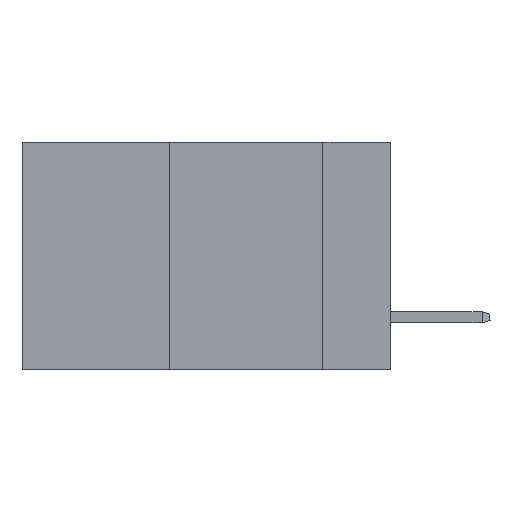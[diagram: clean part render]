
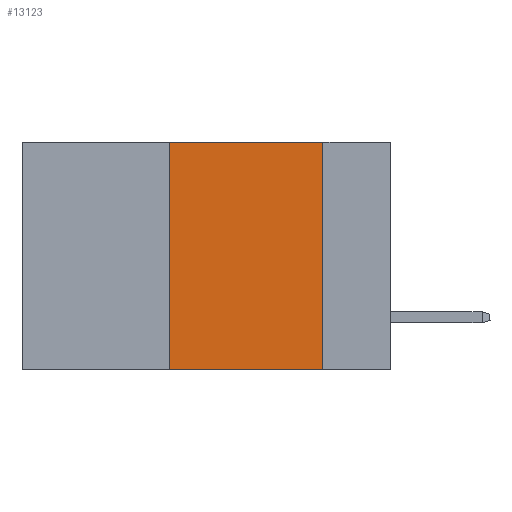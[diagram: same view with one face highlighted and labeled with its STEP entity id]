
A CAD part, left-side view. The second image highlights one B-rep face of the part: STEP entity #13123.
In plain terms, the highlighted planar face has unit normal (-1, 0, 0).
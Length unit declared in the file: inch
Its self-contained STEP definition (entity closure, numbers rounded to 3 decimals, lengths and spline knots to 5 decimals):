
#54 = ORIENTED_EDGE ( 'NONE', *, *, #2807, .F. ) ;
#209 = ORIENTED_EDGE ( 'NONE', *, *, #2925, .T. ) ;
#1054 = VERTEX_POINT ( 'NONE', #7221 ) ;
#1187 = EDGE_CURVE ( 'NONE', #2343, #9184, #7537, .T. ) ;
#1325 = DIRECTION ( 'NONE',  ( 0., -1., 0. ) ) ;
#1524 = CARTESIAN_POINT ( 'NONE',  ( 0., 0.36, 0. ) ) ;
#2074 = CARTESIAN_POINT ( 'NONE',  ( 0., 0.6, 0. ) ) ;
#2343 = VERTEX_POINT ( 'NONE', #8081 ) ;
#2496 = FACE_OUTER_BOUND ( 'NONE', #5296, .T. ) ;
#2801 = LINE ( 'NONE', #4425, #9984 ) ;
#2807 = EDGE_CURVE ( 'NONE', #5415, #2343, #8156, .T. ) ;
#2925 = EDGE_CURVE ( 'NONE', #5415, #1054, #7817, .T. ) ;
#3338 = CARTESIAN_POINT ( 'NONE',  ( 0., 0.6, 0. ) ) ;
#4425 = CARTESIAN_POINT ( 'NONE',  ( 0., 0.11, 0. ) ) ;
#5251 = DIRECTION ( 'NONE',  ( 1., 0., 0. ) ) ;
#5296 = EDGE_LOOP ( 'NONE', ( #10670, #8789, #54, #209 ) ) ;
#5415 = VERTEX_POINT ( 'NONE', #11027 ) ;
#7221 = CARTESIAN_POINT ( 'NONE',  ( 0., 0.11, -0.37 ) ) ;
#7290 = DIRECTION ( 'NONE',  ( 0., 0., -1. ) ) ;
#7537 = LINE ( 'NONE', #3338, #10054 ) ;
#7623 = DIRECTION ( 'NONE',  ( 0., -1., 0. ) ) ;
#7817 = LINE ( 'NONE', #8384, #12337 ) ;
#8081 = CARTESIAN_POINT ( 'NONE',  ( 0., 0.36, 0. ) ) ;
#8156 = LINE ( 'NONE', #1524, #12348 ) ;
#8384 = CARTESIAN_POINT ( 'NONE',  ( 0., 0.6, -0.37 ) ) ;
#8467 = PLANE ( 'NONE',  #8995 ) ;
#8789 = ORIENTED_EDGE ( 'NONE', *, *, #1187, .F. ) ;
#8995 = AXIS2_PLACEMENT_3D ( 'NONE', #2074, #5251, #7290 ) ;
#9184 = VERTEX_POINT ( 'NONE', #10017 ) ;
#9984 = VECTOR ( 'NONE', #10767, 39.37008 ) ;
#10017 = CARTESIAN_POINT ( 'NONE',  ( 0., 0.11, 0. ) ) ;
#10054 = VECTOR ( 'NONE', #1325, 39.37008 ) ;
#10670 = ORIENTED_EDGE ( 'NONE', *, *, #13771, .F. ) ;
#10767 = DIRECTION ( 'NONE',  ( 0., 0., -1. ) ) ;
#11027 = CARTESIAN_POINT ( 'NONE',  ( 0., 0.36, -0.37 ) ) ;
#11171 = DIRECTION ( 'NONE',  ( 0., 0., 1. ) ) ;
#12337 = VECTOR ( 'NONE', #7623, 39.37008 ) ;
#12348 = VECTOR ( 'NONE', #11171, 39.37008 ) ;
#13123 = ADVANCED_FACE ( 'NONE', ( #2496 ), #8467, .F. ) ;
#13771 = EDGE_CURVE ( 'NONE', #9184, #1054, #2801, .T. ) ;
